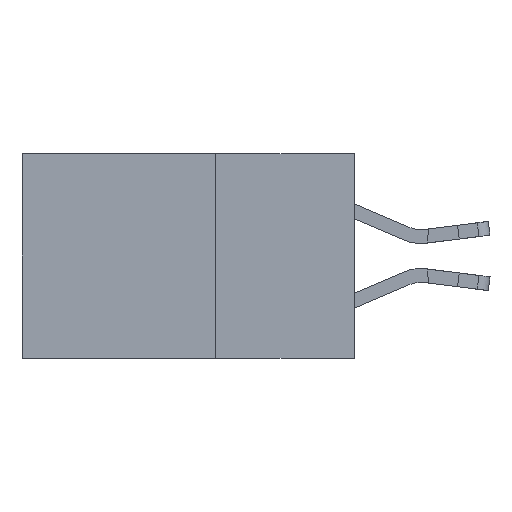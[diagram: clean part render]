
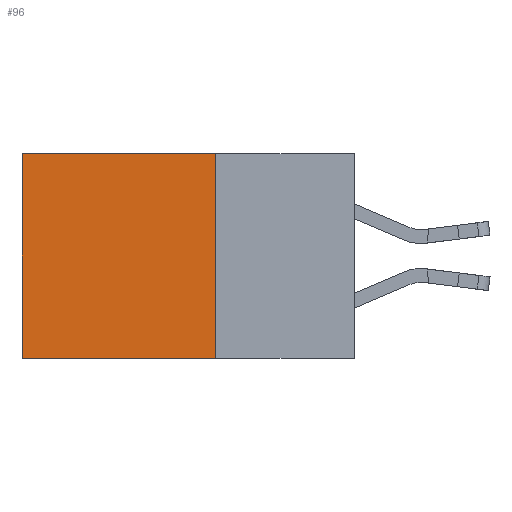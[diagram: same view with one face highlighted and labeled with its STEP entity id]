
A CAD part, left-side view. The second image highlights one B-rep face of the part: STEP entity #96.
In plain terms, the highlighted planar face has unit normal (-1, 0, 0).
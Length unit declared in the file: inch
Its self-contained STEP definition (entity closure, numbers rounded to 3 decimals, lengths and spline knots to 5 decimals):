
#96 = ADVANCED_FACE ( 'NONE', ( #6969 ), #11761, .F. ) ;
#284 = CARTESIAN_POINT ( 'NONE',  ( 0.298, 0.25, 0. ) ) ;
#1940 = EDGE_LOOP ( 'NONE', ( #17375, #16731, #14935, #21486 ) ) ;
#2729 = CARTESIAN_POINT ( 'NONE',  ( 0.298, 0.6, 0. ) ) ;
#3404 = VERTEX_POINT ( 'NONE', #7699 ) ;
#3890 = VERTEX_POINT ( 'NONE', #5255 ) ;
#4970 = AXIS2_PLACEMENT_3D ( 'NONE', #8823, #18937, #6946 ) ;
#5255 = CARTESIAN_POINT ( 'NONE',  ( 0.298, 0.25, -0.37 ) ) ;
#5487 = CARTESIAN_POINT ( 'NONE',  ( 0.298, 0.25, 0. ) ) ;
#6946 = DIRECTION ( 'NONE',  ( 0., 0., -1. ) ) ;
#6969 = FACE_OUTER_BOUND ( 'NONE', #1940, .T. ) ;
#7699 = CARTESIAN_POINT ( 'NONE',  ( 0.298, 0.6, 0. ) ) ;
#7827 = LINE ( 'NONE', #16822, #21430 ) ;
#8227 = VERTEX_POINT ( 'NONE', #5487 ) ;
#8664 = DIRECTION ( 'NONE',  ( 0., 0., -1. ) ) ;
#8823 = CARTESIAN_POINT ( 'NONE',  ( 0.298, 0.25, 0. ) ) ;
#10125 = EDGE_CURVE ( 'NONE', #3890, #19338, #18004, .T. ) ;
#10162 = DIRECTION ( 'NONE',  ( 0., 1., 0. ) ) ;
#11761 = PLANE ( 'NONE',  #4970 ) ;
#12001 = CARTESIAN_POINT ( 'NONE',  ( 0.298, 0.6, -0.37 ) ) ;
#12369 = LINE ( 'NONE', #284, #21108 ) ;
#12457 = LINE ( 'NONE', #2729, #16808 ) ;
#13582 = VECTOR ( 'NONE', #19744, 39.37008 ) ;
#13663 = EDGE_CURVE ( 'NONE', #8227, #3890, #12369, .T. ) ;
#14390 = CARTESIAN_POINT ( 'NONE',  ( 0.298, 0.25, -0.37 ) ) ;
#14935 = ORIENTED_EDGE ( 'NONE', *, *, #13663, .F. ) ;
#16731 = ORIENTED_EDGE ( 'NONE', *, *, #10125, .F. ) ;
#16808 = VECTOR ( 'NONE', #18427, 39.37008 ) ;
#16822 = CARTESIAN_POINT ( 'NONE',  ( 0.298, 0.25, 0. ) ) ;
#17375 = ORIENTED_EDGE ( 'NONE', *, *, #18115, .T. ) ;
#18004 = LINE ( 'NONE', #14390, #13582 ) ;
#18115 = EDGE_CURVE ( 'NONE', #3404, #19338, #12457, .T. ) ;
#18427 = DIRECTION ( 'NONE',  ( 0., 0., -1. ) ) ;
#18683 = EDGE_CURVE ( 'NONE', #8227, #3404, #7827, .T. ) ;
#18937 = DIRECTION ( 'NONE',  ( 1., 0., 0. ) ) ;
#19338 = VERTEX_POINT ( 'NONE', #12001 ) ;
#19744 = DIRECTION ( 'NONE',  ( 0., 1., 0. ) ) ;
#21108 = VECTOR ( 'NONE', #8664, 39.37008 ) ;
#21430 = VECTOR ( 'NONE', #10162, 39.37008 ) ;
#21486 = ORIENTED_EDGE ( 'NONE', *, *, #18683, .T. ) ;
